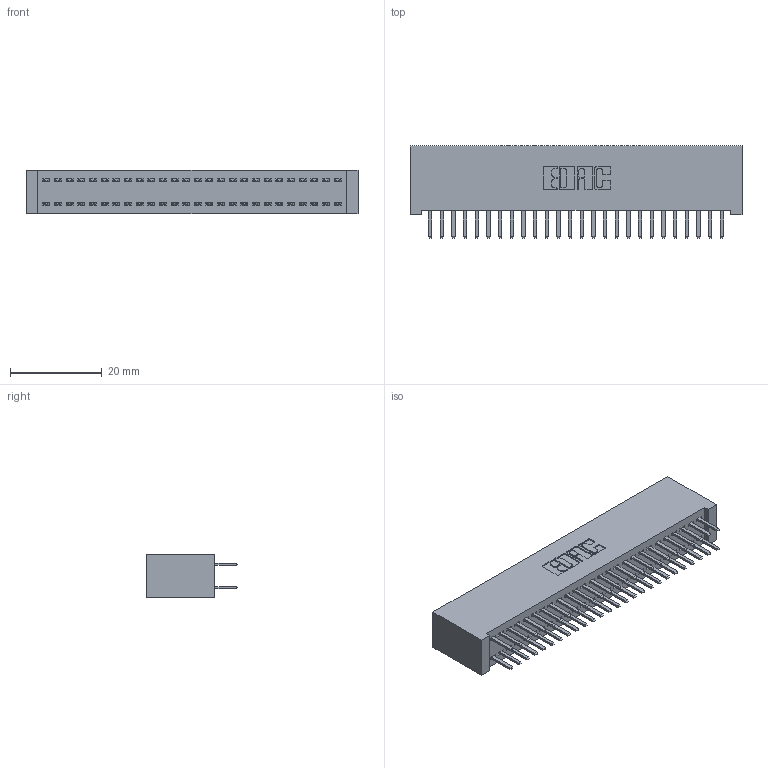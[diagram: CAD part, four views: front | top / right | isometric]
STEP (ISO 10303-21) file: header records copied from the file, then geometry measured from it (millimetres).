
FILE_DESCRIPTION (( 'STEP AP203' ), '1' );
FILE_NAME ('392-052-520-201.STEP', '2019-10-08T12:13:28', ( '' ), ( '' ), 'SwSTEP 2.0', 'SolidWorks 2016', '' );
FILE_SCHEMA (( 'CONFIG_CONTROL_DESIGN' ));
Length unit declared in the file: inch
Products named in the file (3): 342 Part_Lugless; 345-292-001_345-293-120; 392-052-520-201
Assembly tree (53 placements, depth 2):
  392-052-520-201
    342 Part_Lugless
    345-292-001_345-293-120  x52
Bounding box: 72.29 x 20.02 x 9.4 mm (x, y, z)
Volume: 6836 mm3; surface area: 11125.4 mm2
Topology: 53 solids, 53 shells, 3014 faces, 8751 edges, 5694 vertices
Faces by surface type: plane 2038, cylinder 976
Entity records: 18501 total; most frequent: CARTESIAN_POINT 3094, ORIENTED_EDGE 3018, DIRECTION 2653, EDGE_CURVE 1509, VECTOR 1385, LINE 1385, VERTEX_POINT 1002, AXIS2_PLACEMENT_3D 634
